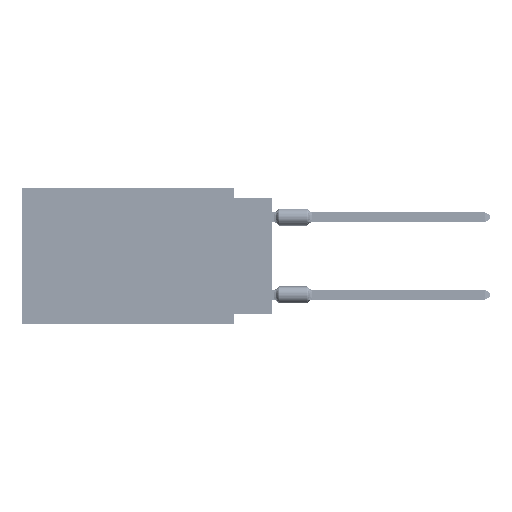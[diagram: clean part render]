
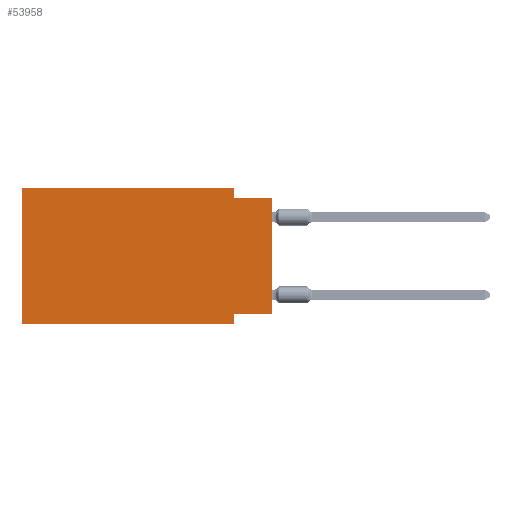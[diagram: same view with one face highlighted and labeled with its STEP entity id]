
A CAD part, left-side view. The second image highlights one B-rep face of the part: STEP entity #53958.
In plain terms, the highlighted planar face has unit normal (-1, 0, 0).
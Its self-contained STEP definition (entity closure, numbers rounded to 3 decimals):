
#202 = VERTEX_POINT ( 'NONE', #68171 ) ;
#786 = CARTESIAN_POINT ( 'NONE',  ( 0., 16.383, -8.89 ) ) ;
#1542 = EDGE_LOOP ( 'NONE', ( #49952, #63873, #11396, #60251, #37698, #19553, #10527, #18099 ) ) ;
#3552 = DIRECTION ( 'NONE',  ( 0., 0., 1. ) ) ;
#3804 = CARTESIAN_POINT ( 'NONE',  ( 0., 2.54, -8.89 ) ) ;
#4337 = VERTEX_POINT ( 'NONE', #21116 ) ;
#7239 = VECTOR ( 'NONE', #66488, 1000. ) ;
#7870 = EDGE_CURVE ( 'NONE', #85283, #15459, #62879, .T. ) ;
#8107 = LINE ( 'NONE', #27216, #76317 ) ;
#8673 = EDGE_CURVE ( 'NONE', #81753, #202, #8107, .T. ) ;
#9172 = DIRECTION ( 'NONE',  ( 0., -1., 0. ) ) ;
#9702 = DIRECTION ( 'NONE',  ( 0., 0., 1. ) ) ;
#10212 = CARTESIAN_POINT ( 'NONE',  ( 0., 0., 0. ) ) ;
#10527 = ORIENTED_EDGE ( 'NONE', *, *, #46836, .F. ) ;
#11396 = ORIENTED_EDGE ( 'NONE', *, *, #8673, .F. ) ;
#11789 = EDGE_CURVE ( 'NONE', #54760, #81753, #58849, .T. ) ;
#12772 = LINE ( 'NONE', #40276, #7239 ) ;
#15459 = VERTEX_POINT ( 'NONE', #3804 ) ;
#18008 = EDGE_CURVE ( 'NONE', #85283, #54760, #75437, .T. ) ;
#18099 = ORIENTED_EDGE ( 'NONE', *, *, #68778, .F. ) ;
#18449 = CARTESIAN_POINT ( 'NONE',  ( 0., 2.54, 0. ) ) ;
#19553 = ORIENTED_EDGE ( 'NONE', *, *, #7870, .T. ) ;
#21116 = CARTESIAN_POINT ( 'NONE',  ( 0., 2.54, -8.255 ) ) ;
#22302 = VECTOR ( 'NONE', #23766, 1000. ) ;
#23766 = DIRECTION ( 'NONE',  ( 0., 0., -1. ) ) ;
#24975 = VERTEX_POINT ( 'NONE', #66460 ) ;
#25485 = VECTOR ( 'NONE', #65942, 1000. ) ;
#26003 = CARTESIAN_POINT ( 'NONE',  ( 0., 16.383, 0. ) ) ;
#27216 = CARTESIAN_POINT ( 'NONE',  ( 0., 2.54, 0. ) ) ;
#28081 = DIRECTION ( 'NONE',  ( 0., 0., -1. ) ) ;
#30047 = VECTOR ( 'NONE', #37156, 1000. ) ;
#33799 = PLANE ( 'NONE',  #65784 ) ;
#37156 = DIRECTION ( 'NONE',  ( 0., -1., 0. ) ) ;
#37698 = ORIENTED_EDGE ( 'NONE', *, *, #18008, .F. ) ;
#40276 = CARTESIAN_POINT ( 'NONE',  ( 0., 0., -8.255 ) ) ;
#41220 = EDGE_CURVE ( 'NONE', #59555, #24975, #71015, .T. ) ;
#44167 = CARTESIAN_POINT ( 'NONE',  ( 0., 2.54, -8.89 ) ) ;
#46836 = EDGE_CURVE ( 'NONE', #4337, #15459, #69058, .T. ) ;
#49952 = ORIENTED_EDGE ( 'NONE', *, *, #41220, .T. ) ;
#52635 = EDGE_CURVE ( 'NONE', #202, #24975, #83773, .T. ) ;
#52764 = CARTESIAN_POINT ( 'NONE',  ( 0., 16.383, -8.89 ) ) ;
#52899 = DIRECTION ( 'NONE',  ( 0., 0., -1. ) ) ;
#53958 = ADVANCED_FACE ( 'NONE', ( #59563 ), #33799, .F. ) ;
#54760 = VERTEX_POINT ( 'NONE', #80971 ) ;
#57817 = VECTOR ( 'NONE', #9172, 1000. ) ;
#58849 = LINE ( 'NONE', #26003, #25485 ) ;
#59555 = VERTEX_POINT ( 'NONE', #69759 ) ;
#59563 = FACE_OUTER_BOUND ( 'NONE', #1542, .T. ) ;
#60251 = ORIENTED_EDGE ( 'NONE', *, *, #11789, .F. ) ;
#62879 = LINE ( 'NONE', #786, #57817 ) ;
#63873 = ORIENTED_EDGE ( 'NONE', *, *, #52635, .F. ) ;
#65784 = AXIS2_PLACEMENT_3D ( 'NONE', #74642, #73318, #52899 ) ;
#65942 = DIRECTION ( 'NONE',  ( 0., -1., 0. ) ) ;
#66460 = CARTESIAN_POINT ( 'NONE',  ( 0., 0., -0.635 ) ) ;
#66488 = DIRECTION ( 'NONE',  ( 0., 1., 0. ) ) ;
#68171 = CARTESIAN_POINT ( 'NONE',  ( 0., 2.54, -0.635 ) ) ;
#68778 = EDGE_CURVE ( 'NONE', #59555, #4337, #12772, .T. ) ;
#69058 = LINE ( 'NONE', #44167, #22302 ) ;
#69633 = CARTESIAN_POINT ( 'NONE',  ( 0., 16.383, 0. ) ) ;
#69759 = CARTESIAN_POINT ( 'NONE',  ( 0., 0., -8.255 ) ) ;
#71015 = LINE ( 'NONE', #10212, #79911 ) ;
#73318 = DIRECTION ( 'NONE',  ( 1., 0., 0. ) ) ;
#73541 = VECTOR ( 'NONE', #9702, 1000. ) ;
#74642 = CARTESIAN_POINT ( 'NONE',  ( 0., 16.383, 0. ) ) ;
#75437 = LINE ( 'NONE', #69633, #73541 ) ;
#76317 = VECTOR ( 'NONE', #28081, 1000. ) ;
#79911 = VECTOR ( 'NONE', #3552, 1000. ) ;
#80971 = CARTESIAN_POINT ( 'NONE',  ( 0., 16.383, 0. ) ) ;
#81753 = VERTEX_POINT ( 'NONE', #18449 ) ;
#83336 = CARTESIAN_POINT ( 'NONE',  ( 0., 0., -0.635 ) ) ;
#83773 = LINE ( 'NONE', #83336, #30047 ) ;
#85283 = VERTEX_POINT ( 'NONE', #52764 ) ;
